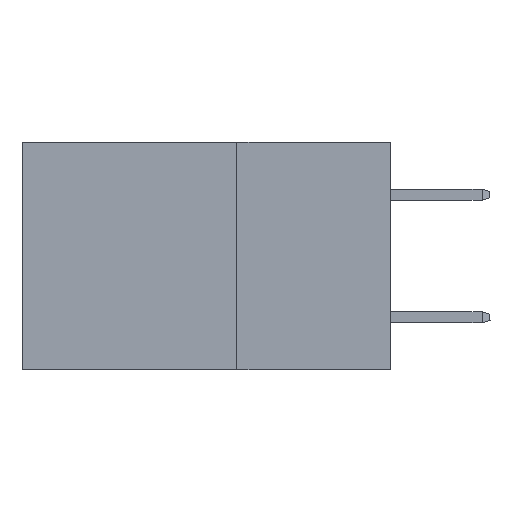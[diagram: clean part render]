
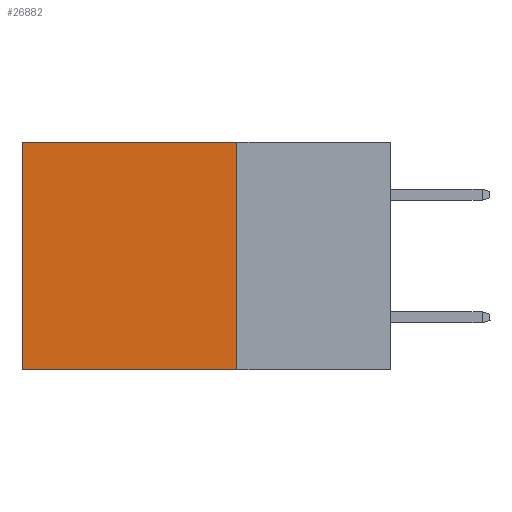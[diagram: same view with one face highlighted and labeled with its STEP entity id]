
A CAD part, left-side view. The second image highlights one B-rep face of the part: STEP entity #26882.
In plain terms, the highlighted planar face has unit normal (-1, 0, 0).
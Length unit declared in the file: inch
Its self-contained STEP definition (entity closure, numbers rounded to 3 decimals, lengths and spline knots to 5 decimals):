
#522 = ORIENTED_EDGE ( 'NONE', *, *, #24234, .T. ) ;
#1366 = CARTESIAN_POINT ( 'NONE',  ( 0.2875, 0.25, 0. ) ) ;
#1701 = LINE ( 'NONE', #22204, #25734 ) ;
#2063 = ORIENTED_EDGE ( 'NONE', *, *, #19536, .T. ) ;
#2111 = CARTESIAN_POINT ( 'NONE',  ( 0.2875, 0.25, 0. ) ) ;
#2456 = FACE_OUTER_BOUND ( 'NONE', #31270, .T. ) ;
#3429 = VECTOR ( 'NONE', #11396, 39.37008 ) ;
#3528 = LINE ( 'NONE', #31488, #29803 ) ;
#4889 = CARTESIAN_POINT ( 'NONE',  ( 0.2875, 0.6, 0. ) ) ;
#7366 = DIRECTION ( 'NONE',  ( 1., 0., 0. ) ) ;
#8373 = CARTESIAN_POINT ( 'NONE',  ( 0.2875, 0.25, -0.37 ) ) ;
#9214 = CARTESIAN_POINT ( 'NONE',  ( 0.2875, 0.6, 0. ) ) ;
#11231 = CARTESIAN_POINT ( 'NONE',  ( 0.2875, 0.25, -0.37 ) ) ;
#11396 = DIRECTION ( 'NONE',  ( 0., 1., 0. ) ) ;
#12018 = ORIENTED_EDGE ( 'NONE', *, *, #33118, .F. ) ;
#14887 = EDGE_CURVE ( 'NONE', #27649, #16135, #1701, .T. ) ;
#15501 = PLANE ( 'NONE',  #32006 ) ;
#16135 = VERTEX_POINT ( 'NONE', #8373 ) ;
#16987 = ORIENTED_EDGE ( 'NONE', *, *, #14887, .F. ) ;
#17178 = VECTOR ( 'NONE', #19562, 39.37008 ) ;
#19536 = EDGE_CURVE ( 'NONE', #24176, #31757, #27533, .T. ) ;
#19562 = DIRECTION ( 'NONE',  ( 0., 0., -1. ) ) ;
#19677 = DIRECTION ( 'NONE',  ( 0., 0., -1. ) ) ;
#22022 = CARTESIAN_POINT ( 'NONE',  ( 0.2875, 0.6, -0.37 ) ) ;
#22204 = CARTESIAN_POINT ( 'NONE',  ( 0.2875, 0.25, 0. ) ) ;
#24176 = VERTEX_POINT ( 'NONE', #4889 ) ;
#24234 = EDGE_CURVE ( 'NONE', #27649, #24176, #3528, .T. ) ;
#24452 = LINE ( 'NONE', #11231, #3429 ) ;
#25734 = VECTOR ( 'NONE', #19677, 39.37008 ) ;
#25845 = DIRECTION ( 'NONE',  ( 0., 0., -1. ) ) ;
#26420 = DIRECTION ( 'NONE',  ( 0., 1., 0. ) ) ;
#26882 = ADVANCED_FACE ( 'NONE', ( #2456 ), #15501, .F. ) ;
#27533 = LINE ( 'NONE', #9214, #17178 ) ;
#27649 = VERTEX_POINT ( 'NONE', #1366 ) ;
#29803 = VECTOR ( 'NONE', #26420, 39.37008 ) ;
#31270 = EDGE_LOOP ( 'NONE', ( #2063, #12018, #16987, #522 ) ) ;
#31488 = CARTESIAN_POINT ( 'NONE',  ( 0.2875, 0.25, 0. ) ) ;
#31757 = VERTEX_POINT ( 'NONE', #22022 ) ;
#32006 = AXIS2_PLACEMENT_3D ( 'NONE', #2111, #7366, #25845 ) ;
#33118 = EDGE_CURVE ( 'NONE', #16135, #31757, #24452, .T. ) ;
